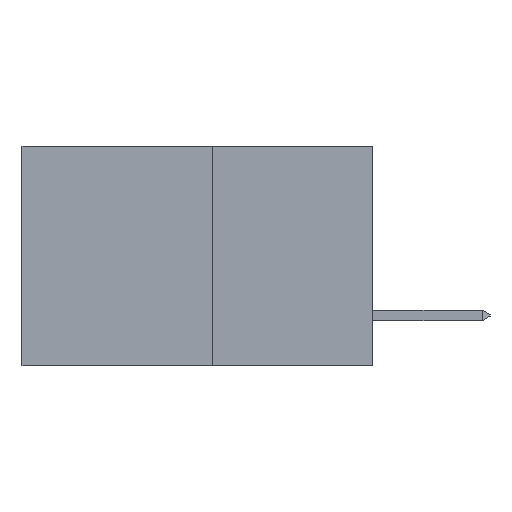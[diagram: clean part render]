
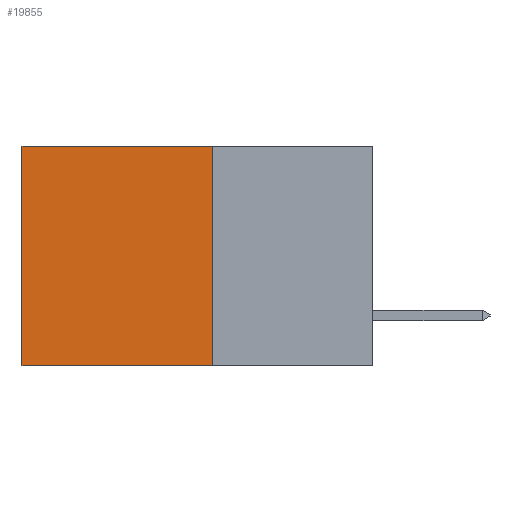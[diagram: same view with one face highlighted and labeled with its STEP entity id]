
A CAD part, left-side view. The second image highlights one B-rep face of the part: STEP entity #19855.
In plain terms, the highlighted planar face has unit normal (-1, 0, 0).
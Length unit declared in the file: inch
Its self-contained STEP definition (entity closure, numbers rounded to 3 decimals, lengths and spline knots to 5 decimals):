
#536 = LINE ( 'NONE', #11344, #16932 ) ;
#1403 = CARTESIAN_POINT ( 'NONE',  ( 0.277, 0.59, -0.37 ) ) ;
#1537 = EDGE_CURVE ( 'NONE', #11742, #8495, #14523, .T. ) ;
#1834 = VECTOR ( 'NONE', #2591, 39.37008 ) ;
#2011 = VERTEX_POINT ( 'NONE', #17870 ) ;
#2591 = DIRECTION ( 'NONE',  ( 0., 1., 0. ) ) ;
#3000 = DIRECTION ( 'NONE',  ( 1., 0., 0. ) ) ;
#3163 = ORIENTED_EDGE ( 'NONE', *, *, #12367, .T. ) ;
#3270 = AXIS2_PLACEMENT_3D ( 'NONE', #12557, #3000, #14147 ) ;
#3651 = CARTESIAN_POINT ( 'NONE',  ( 0.277, 0.59, -0.37 ) ) ;
#5179 = EDGE_CURVE ( 'NONE', #9450, #11742, #536, .T. ) ;
#5693 = CARTESIAN_POINT ( 'NONE',  ( 0.277, 0.27, 0. ) ) ;
#5975 = EDGE_LOOP ( 'NONE', ( #3163, #11047, #17565, #11644 ) ) ;
#6756 = LINE ( 'NONE', #1403, #14777 ) ;
#8495 = VERTEX_POINT ( 'NONE', #3651 ) ;
#9450 = VERTEX_POINT ( 'NONE', #11375 ) ;
#10214 = CARTESIAN_POINT ( 'NONE',  ( 0.277, 0.27, -0.37 ) ) ;
#10940 = PLANE ( 'NONE',  #3270 ) ;
#11047 = ORIENTED_EDGE ( 'NONE', *, *, #1537, .F. ) ;
#11344 = CARTESIAN_POINT ( 'NONE',  ( 0.277, 0.27, -0.37 ) ) ;
#11375 = CARTESIAN_POINT ( 'NONE',  ( 0.277, 0.27, 0. ) ) ;
#11644 = ORIENTED_EDGE ( 'NONE', *, *, #11730, .T. ) ;
#11730 = EDGE_CURVE ( 'NONE', #9450, #2011, #14552, .T. ) ;
#11742 = VERTEX_POINT ( 'NONE', #18487 ) ;
#11971 = DIRECTION ( 'NONE',  ( 0., 0., -1. ) ) ;
#11978 = FACE_OUTER_BOUND ( 'NONE', #5975, .T. ) ;
#12367 = EDGE_CURVE ( 'NONE', #2011, #8495, #6756, .T. ) ;
#12557 = CARTESIAN_POINT ( 'NONE',  ( 0.277, 0.27, -0.37 ) ) ;
#14147 = DIRECTION ( 'NONE',  ( 0., 0., -1. ) ) ;
#14523 = LINE ( 'NONE', #10214, #18699 ) ;
#14552 = LINE ( 'NONE', #5693, #1834 ) ;
#14777 = VECTOR ( 'NONE', #17296, 39.37008 ) ;
#16932 = VECTOR ( 'NONE', #11971, 39.37008 ) ;
#17296 = DIRECTION ( 'NONE',  ( 0., 0., -1. ) ) ;
#17565 = ORIENTED_EDGE ( 'NONE', *, *, #5179, .F. ) ;
#17870 = CARTESIAN_POINT ( 'NONE',  ( 0.277, 0.59, 0. ) ) ;
#18370 = DIRECTION ( 'NONE',  ( 0., 1., 0. ) ) ;
#18487 = CARTESIAN_POINT ( 'NONE',  ( 0.277, 0.27, -0.37 ) ) ;
#18699 = VECTOR ( 'NONE', #18370, 39.37008 ) ;
#19855 = ADVANCED_FACE ( 'NONE', ( #11978 ), #10940, .F. ) ;
